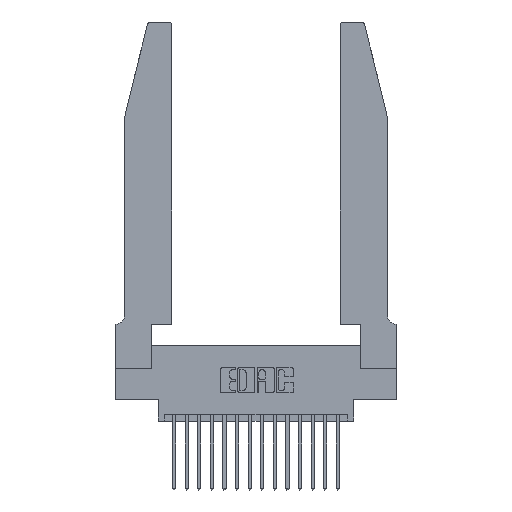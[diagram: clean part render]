
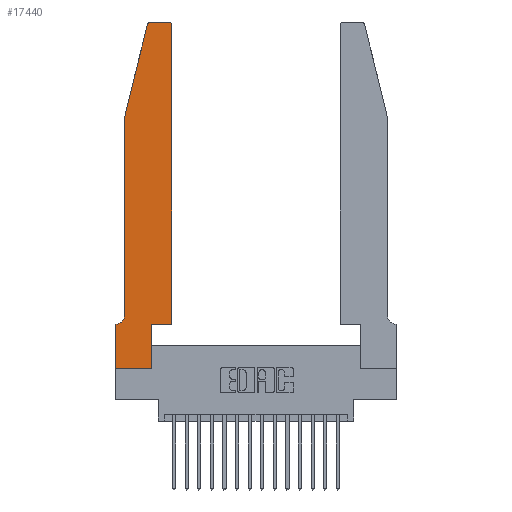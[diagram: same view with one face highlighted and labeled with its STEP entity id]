
A CAD part, top view. The second image highlights one B-rep face of the part: STEP entity #17440.
In plain terms, the highlighted planar face has unit normal (0, 0, 1).
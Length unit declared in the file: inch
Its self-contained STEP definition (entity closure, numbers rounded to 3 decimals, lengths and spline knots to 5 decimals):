
#93 = VECTOR ( 'NONE', #415, 39.37008 ) ;
#179 = FACE_OUTER_BOUND ( 'NONE', #6854, .T. ) ;
#285 = AXIS2_PLACEMENT_3D ( 'NONE', #17689, #4054, #10205 ) ;
#415 = DIRECTION ( 'NONE',  ( -1., 0., 0. ) ) ;
#453 = EDGE_CURVE ( 'NONE', #8301, #5451, #3191, .T. ) ;
#562 = VERTEX_POINT ( 'NONE', #9286 ) ;
#695 = VERTEX_POINT ( 'NONE', #16188 ) ;
#1135 = CARTESIAN_POINT ( 'NONE',  ( 0.284, 2.72, 0.37 ) ) ;
#1946 = CARTESIAN_POINT ( 'NONE',  ( 0.2865, 0., 0.37 ) ) ;
#1969 = LINE ( 'NONE', #16452, #17612 ) ;
#2007 = EDGE_CURVE ( 'NONE', #19103, #562, #1969, .T. ) ;
#2160 = ORIENTED_EDGE ( 'NONE', *, *, #15484, .T. ) ;
#2177 = CARTESIAN_POINT ( 'NONE',  ( 0.4205, 2.72, 0.37 ) ) ;
#2367 = VERTEX_POINT ( 'NONE', #12789 ) ;
#2908 = VERTEX_POINT ( 'NONE', #9650 ) ;
#3191 = LINE ( 'NONE', #12566, #93 ) ;
#3327 = VECTOR ( 'NONE', #10907, 39.37008 ) ;
#3646 = CIRCLE ( 'NONE', #9320, 0.03 ) ;
#4035 = LINE ( 'NONE', #5702, #4755 ) ;
#4052 = DIRECTION ( 'NONE',  ( -0.239, -0.971, 0. ) ) ;
#4054 = DIRECTION ( 'NONE',  ( 0., 0., 1. ) ) ;
#4059 = AXIS2_PLACEMENT_3D ( 'NONE', #17231, #8950, #10615 ) ;
#4704 = ORIENTED_EDGE ( 'NONE', *, *, #6034, .T. ) ;
#4755 = VECTOR ( 'NONE', #14889, 39.37008 ) ;
#5200 = ORIENTED_EDGE ( 'NONE', *, *, #18867, .T. ) ;
#5451 = VERTEX_POINT ( 'NONE', #17337 ) ;
#5698 = ORIENTED_EDGE ( 'NONE', *, *, #8752, .T. ) ;
#5702 = CARTESIAN_POINT ( 'NONE',  ( 0., 0., 0.37 ) ) ;
#6034 = EDGE_CURVE ( 'NONE', #8106, #695, #7501, .T. ) ;
#6265 = DIRECTION ( 'NONE',  ( 0., 0., 1. ) ) ;
#6612 = CARTESIAN_POINT ( 'NONE',  ( 0.0755, 2., 0.37 ) ) ;
#6854 = EDGE_LOOP ( 'NONE', ( #8631, #5200, #10149, #2160, #4704, #8794, #18856, #8774, #5698, #8565, #11185, #12308 ) ) ;
#7501 = CIRCLE ( 'NONE', #4059, 0.07 ) ;
#7561 = LINE ( 'NONE', #15207, #9487 ) ;
#7913 = LINE ( 'NONE', #16632, #11276 ) ;
#8106 = VERTEX_POINT ( 'NONE', #10692 ) ;
#8137 = AXIS2_PLACEMENT_3D ( 'NONE', #2177, #6265, #12407 ) ;
#8174 = EDGE_CURVE ( 'NONE', #15704, #19103, #15984, .T. ) ;
#8301 = VERTEX_POINT ( 'NONE', #17362 ) ;
#8553 = DIRECTION ( 'NONE',  ( 0., 0., 1. ) ) ;
#8565 = ORIENTED_EDGE ( 'NONE', *, *, #8174, .T. ) ;
#8595 = CARTESIAN_POINT ( 'NONE',  ( 0.0755, 2., 0.37 ) ) ;
#8631 = ORIENTED_EDGE ( 'NONE', *, *, #453, .T. ) ;
#8752 = EDGE_CURVE ( 'NONE', #13152, #15704, #7913, .T. ) ;
#8774 = ORIENTED_EDGE ( 'NONE', *, *, #10874, .T. ) ;
#8794 = ORIENTED_EDGE ( 'NONE', *, *, #16267, .T. ) ;
#8950 = DIRECTION ( 'NONE',  ( 0., 0., -1. ) ) ;
#9163 = CARTESIAN_POINT ( 'NONE',  ( 0., 0., 0.37 ) ) ;
#9286 = CARTESIAN_POINT ( 'NONE',  ( 0.4505, 2.72, 0.37 ) ) ;
#9320 = AXIS2_PLACEMENT_3D ( 'NONE', #1135, #8553, #19308 ) ;
#9360 = VERTEX_POINT ( 'NONE', #10822 ) ;
#9487 = VECTOR ( 'NONE', #11928, 39.37008 ) ;
#9650 = CARTESIAN_POINT ( 'NONE',  ( 0., 0., 0.37 ) ) ;
#10149 = ORIENTED_EDGE ( 'NONE', *, *, #13855, .T. ) ;
#10205 = DIRECTION ( 'NONE',  ( 1., 0., 0. ) ) ;
#10594 = VECTOR ( 'NONE', #4052, 39.37008 ) ;
#10615 = DIRECTION ( 'NONE',  ( -1., 0., 0. ) ) ;
#10692 = CARTESIAN_POINT ( 'NONE',  ( 0.0755, 0.42, 0.37 ) ) ;
#10779 = EDGE_CURVE ( 'NONE', #2367, #2908, #4035, .T. ) ;
#10822 = CARTESIAN_POINT ( 'NONE',  ( 0.0755, 2., 0.37 ) ) ;
#10874 = EDGE_CURVE ( 'NONE', #2908, #13152, #19011, .T. ) ;
#10907 = DIRECTION ( 'NONE',  ( 1., 0., 0. ) ) ;
#11185 = ORIENTED_EDGE ( 'NONE', *, *, #2007, .T. ) ;
#11243 = VECTOR ( 'NONE', #15606, 39.37008 ) ;
#11276 = VECTOR ( 'NONE', #18079, 39.37008 ) ;
#11928 = DIRECTION ( 'NONE',  ( -1., 0., 0. ) ) ;
#12308 = ORIENTED_EDGE ( 'NONE', *, *, #13632, .T. ) ;
#12407 = DIRECTION ( 'NONE',  ( 1., 0., 0. ) ) ;
#12566 = CARTESIAN_POINT ( 'NONE',  ( 0.2605, 2.75, 0.37 ) ) ;
#12579 = CARTESIAN_POINT ( 'NONE',  ( 0.25487, 2.72718, 0.37 ) ) ;
#12789 = CARTESIAN_POINT ( 'NONE',  ( 0., 0.35, 0.37 ) ) ;
#13119 = PLANE ( 'NONE',  #285 ) ;
#13152 = VERTEX_POINT ( 'NONE', #1946 ) ;
#13632 = EDGE_CURVE ( 'NONE', #562, #8301, #14883, .T. ) ;
#13650 = DIRECTION ( 'NONE',  ( 0., 1., 0. ) ) ;
#13855 = EDGE_CURVE ( 'NONE', #18257, #9360, #14152, .T. ) ;
#14061 = CARTESIAN_POINT ( 'NONE',  ( 0.4505, 0.35, 0.37 ) ) ;
#14152 = LINE ( 'NONE', #8595, #10594 ) ;
#14330 = DIRECTION ( 'NONE',  ( 0., -1., 0. ) ) ;
#14883 = CIRCLE ( 'NONE', #8137, 0.03 ) ;
#14889 = DIRECTION ( 'NONE',  ( 0., -1., 0. ) ) ;
#15207 = CARTESIAN_POINT ( 'NONE',  ( 0.0755, 0.35, 0.37 ) ) ;
#15226 = CARTESIAN_POINT ( 'NONE',  ( 0.2865, 0.35, 0.37 ) ) ;
#15484 = EDGE_CURVE ( 'NONE', #9360, #8106, #15698, .T. ) ;
#15606 = DIRECTION ( 'NONE',  ( 1., 0., 0. ) ) ;
#15698 = LINE ( 'NONE', #6612, #17331 ) ;
#15704 = VERTEX_POINT ( 'NONE', #15226 ) ;
#15984 = LINE ( 'NONE', #14061, #11243 ) ;
#16188 = CARTESIAN_POINT ( 'NONE',  ( 0.0055, 0.35, 0.37 ) ) ;
#16267 = EDGE_CURVE ( 'NONE', #695, #2367, #7561, .T. ) ;
#16452 = CARTESIAN_POINT ( 'NONE',  ( 0.4505, 0.35, 0.37 ) ) ;
#16632 = CARTESIAN_POINT ( 'NONE',  ( 0.2865, 0.35, 0.37 ) ) ;
#17231 = CARTESIAN_POINT ( 'NONE',  ( 0.0055, 0.42, 0.37 ) ) ;
#17331 = VECTOR ( 'NONE', #14330, 39.37008 ) ;
#17337 = CARTESIAN_POINT ( 'NONE',  ( 0.284, 2.75, 0.37 ) ) ;
#17362 = CARTESIAN_POINT ( 'NONE',  ( 0.4205, 2.75, 0.37 ) ) ;
#17440 = ADVANCED_FACE ( 'NONE', ( #179 ), #13119, .T. ) ;
#17612 = VECTOR ( 'NONE', #13650, 39.37008 ) ;
#17689 = CARTESIAN_POINT ( 'NONE',  ( 0., 0.35, 0.37 ) ) ;
#18079 = DIRECTION ( 'NONE',  ( 0., 1., 0. ) ) ;
#18257 = VERTEX_POINT ( 'NONE', #12579 ) ;
#18856 = ORIENTED_EDGE ( 'NONE', *, *, #10779, .T. ) ;
#18867 = EDGE_CURVE ( 'NONE', #5451, #18257, #3646, .T. ) ;
#19011 = LINE ( 'NONE', #9163, #3327 ) ;
#19103 = VERTEX_POINT ( 'NONE', #19653 ) ;
#19308 = DIRECTION ( 'NONE',  ( 1., 0., 0. ) ) ;
#19653 = CARTESIAN_POINT ( 'NONE',  ( 0.4505, 0.35, 0.37 ) ) ;
